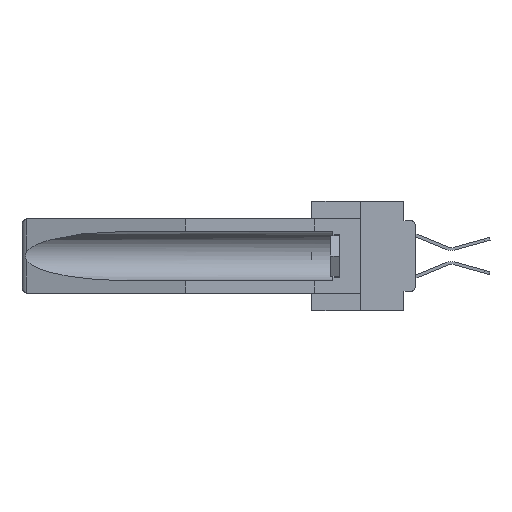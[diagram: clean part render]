
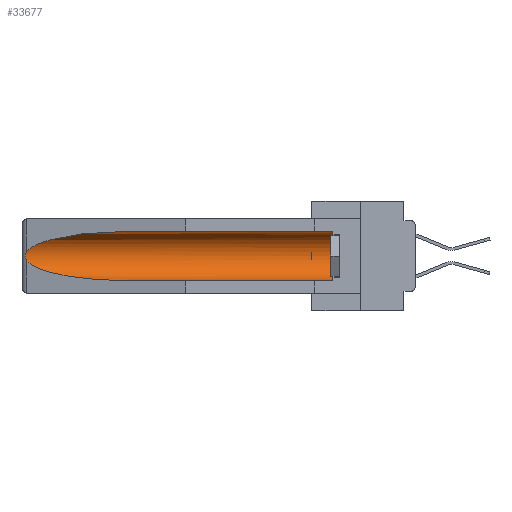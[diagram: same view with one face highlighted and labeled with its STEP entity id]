
A CAD part, left-side view. The second image highlights one B-rep face of the part: STEP entity #33677.
In plain terms, the highlighted cylindrical face has radius 2.857 mm (diameter 5.715 mm), a partial arc.
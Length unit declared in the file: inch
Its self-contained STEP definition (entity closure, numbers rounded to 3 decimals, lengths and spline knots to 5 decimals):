
#136 = CARTESIAN_POINT ( 'NONE',  ( 0.21114, 1.30732, -0.059 ) ) ;
#741 = CARTESIAN_POINT ( 'NONE',  ( 0.155, 0.126, -0.1715 ) ) ;
#966 = CARTESIAN_POINT ( 'NONE',  ( 0.26597, 1.5296, -0.19026 ) ) ;
#1317 = CARTESIAN_POINT ( 'NONE',  ( 0.25451, 1.48313, -0.24835 ) ) ;
#3089 = ORIENTED_EDGE ( 'NONE', *, *, #18745, .T. ) ;
#3515 = CIRCLE ( 'NONE', #35640, 0.1125 ) ;
#3901 = CARTESIAN_POINT ( 'NONE',  ( 0.26537, 1.52718, -0.19328 ) ) ;
#5238 = CYLINDRICAL_SURFACE ( 'NONE', #29683, 0.1125 ) ;
#5448 = VERTEX_POINT ( 'NONE', #33844 ) ;
#6351 = LINE ( 'NONE', #13394, #29406 ) ;
#6737 = CARTESIAN_POINT ( 'NONE',  ( 0.155, 1.07973, -0.059 ) ) ;
#6873 = CARTESIAN_POINT ( 'NONE',  ( 0.26537, 1.52718, -0.14972 ) ) ;
#7442 = CARTESIAN_POINT ( 'NONE',  ( 0.26654, 1.53092, -0.15636 ) ) ;
#8140 =( BOUNDED_CURVE ( )  B_SPLINE_CURVE ( 3, ( #6737, #136, #9704, #32347 ),
 .UNSPECIFIED., .F., .F. ) 
 B_SPLINE_CURVE_WITH_KNOTS ( ( 4, 4 ),
 ( 4.71239, 6.08839 ),
 .UNSPECIFIED. ) 
 CURVE ( )  GEOMETRIC_REPRESENTATION_ITEM ( )  RATIONAL_B_SPLINE_CURVE ( ( 1., 0.848, 0.848, 1. ) ) 
 REPRESENTATION_ITEM ( '' )  );
#8391 = CARTESIAN_POINT ( 'NONE',  ( 0.26537, 1.52718, -0.14972 ) ) ;
#8630 = CARTESIAN_POINT ( 'NONE',  ( 0.21114, 1.30732, -0.284 ) ) ;
#8870 = LINE ( 'NONE', #28832, #24907 ) ;
#9704 = CARTESIAN_POINT ( 'NONE',  ( 0.25451, 1.48313, -0.09465 ) ) ;
#9718 = CARTESIAN_POINT ( 'NONE',  ( 0.155, 0.126, -0.059 ) ) ;
#10705 =( BOUNDED_CURVE ( )  B_SPLINE_CURVE ( 3, ( #36427, #1317, #8630, #15192 ),
 .UNSPECIFIED., .F., .F. ) 
 B_SPLINE_CURVE_WITH_KNOTS ( ( 4, 4 ),
 ( 0.1948, 1.5708 ),
 .UNSPECIFIED. ) 
 CURVE ( )  GEOMETRIC_REPRESENTATION_ITEM ( )  RATIONAL_B_SPLINE_CURVE ( ( 1., 0.848, 0.848, 1. ) ) 
 REPRESENTATION_ITEM ( '' )  );
#11446 = EDGE_CURVE ( 'NONE', #41206, #30749, #16327, .T. ) ;
#12683 = EDGE_CURVE ( 'NONE', #16533, #31933, #3515, .T. ) ;
#13394 = CARTESIAN_POINT ( 'NONE',  ( 0.155, -0.30754, -0.284 ) ) ;
#13444 = CARTESIAN_POINT ( 'NONE',  ( 0.2675, 1.53308, -0.17534 ) ) ;
#15192 = CARTESIAN_POINT ( 'NONE',  ( 0.155, 1.07973, -0.284 ) ) ;
#16262 = ORIENTED_EDGE ( 'NONE', *, *, #23727, .T. ) ;
#16327 = B_SPLINE_CURVE_WITH_KNOTS ( 'NONE', 3,
 ( #6873, #20041, #7442, #39168, #39298, #13444, #16570, #39442, #966, #3901 ),
 .UNSPECIFIED., .F., .F.,
 ( 4, 2, 2, 2, 4 ),
 ( 0., 0.00029, 0.00058, 0.00087, 0.00117 ),
 .UNSPECIFIED. ) ;
#16533 = VERTEX_POINT ( 'NONE', #21623 ) ;
#16570 = CARTESIAN_POINT ( 'NONE',  ( 0.2673, 1.53269, -0.17917 ) ) ;
#17532 = ORIENTED_EDGE ( 'NONE', *, *, #34344, .T. ) ;
#17662 = DIRECTION ( 'NONE',  ( 0., 1., 0. ) ) ;
#18745 = EDGE_CURVE ( 'NONE', #30749, #19804, #10705, .T. ) ;
#19804 = VERTEX_POINT ( 'NONE', #25911 ) ;
#20041 = CARTESIAN_POINT ( 'NONE',  ( 0.26597, 1.52961, -0.15275 ) ) ;
#21623 = CARTESIAN_POINT ( 'NONE',  ( 0.155, 0.126, -0.284 ) ) ;
#22005 = EDGE_LOOP ( 'NONE', ( #17532, #36219, #3089, #28887, #28281, #16262 ) ) ;
#23727 = EDGE_CURVE ( 'NONE', #31933, #5448, #8870, .T. ) ;
#24907 = VECTOR ( 'NONE', #35368, 39.37008 ) ;
#25911 = CARTESIAN_POINT ( 'NONE',  ( 0.155, 1.07973, -0.284 ) ) ;
#26816 = DIRECTION ( 'NONE',  ( 0., -1., 0. ) ) ;
#28281 = ORIENTED_EDGE ( 'NONE', *, *, #12683, .T. ) ;
#28832 = CARTESIAN_POINT ( 'NONE',  ( 0.155, -0.30754, -0.059 ) ) ;
#28887 = ORIENTED_EDGE ( 'NONE', *, *, #36145, .F. ) ;
#29406 = VECTOR ( 'NONE', #35485, 39.37008 ) ;
#29683 = AXIS2_PLACEMENT_3D ( 'NONE', #37174, #17662, #31180 ) ;
#30749 = VERTEX_POINT ( 'NONE', #39589 ) ;
#31180 = DIRECTION ( 'NONE',  ( 0., 0., 1. ) ) ;
#31933 = VERTEX_POINT ( 'NONE', #9718 ) ;
#32347 = CARTESIAN_POINT ( 'NONE',  ( 0.26537, 1.52718, -0.14972 ) ) ;
#33677 = ADVANCED_FACE ( 'NONE', ( #40745 ), #5238, .F. ) ;
#33844 = CARTESIAN_POINT ( 'NONE',  ( 0.155, 1.07973, -0.059 ) ) ;
#34344 = EDGE_CURVE ( 'NONE', #5448, #41206, #8140, .T. ) ;
#35368 = DIRECTION ( 'NONE',  ( 0., 1., 0. ) ) ;
#35485 = DIRECTION ( 'NONE',  ( 0., 1., 0. ) ) ;
#35640 = AXIS2_PLACEMENT_3D ( 'NONE', #741, #26816, #39639 ) ;
#36145 = EDGE_CURVE ( 'NONE', #16533, #19804, #6351, .T. ) ;
#36219 = ORIENTED_EDGE ( 'NONE', *, *, #11446, .T. ) ;
#36427 = CARTESIAN_POINT ( 'NONE',  ( 0.26537, 1.52718, -0.19328 ) ) ;
#37174 = CARTESIAN_POINT ( 'NONE',  ( 0.155, -0.30754, -0.1715 ) ) ;
#39168 = CARTESIAN_POINT ( 'NONE',  ( 0.2673, 1.5327, -0.16383 ) ) ;
#39298 = CARTESIAN_POINT ( 'NONE',  ( 0.2675, 1.53308, -0.16763 ) ) ;
#39442 = CARTESIAN_POINT ( 'NONE',  ( 0.26655, 1.53094, -0.18657 ) ) ;
#39589 = CARTESIAN_POINT ( 'NONE',  ( 0.26537, 1.52718, -0.19328 ) ) ;
#39639 = DIRECTION ( 'NONE',  ( 0., 0., 1. ) ) ;
#40745 = FACE_OUTER_BOUND ( 'NONE', #22005, .T. ) ;
#41206 = VERTEX_POINT ( 'NONE', #8391 ) ;
